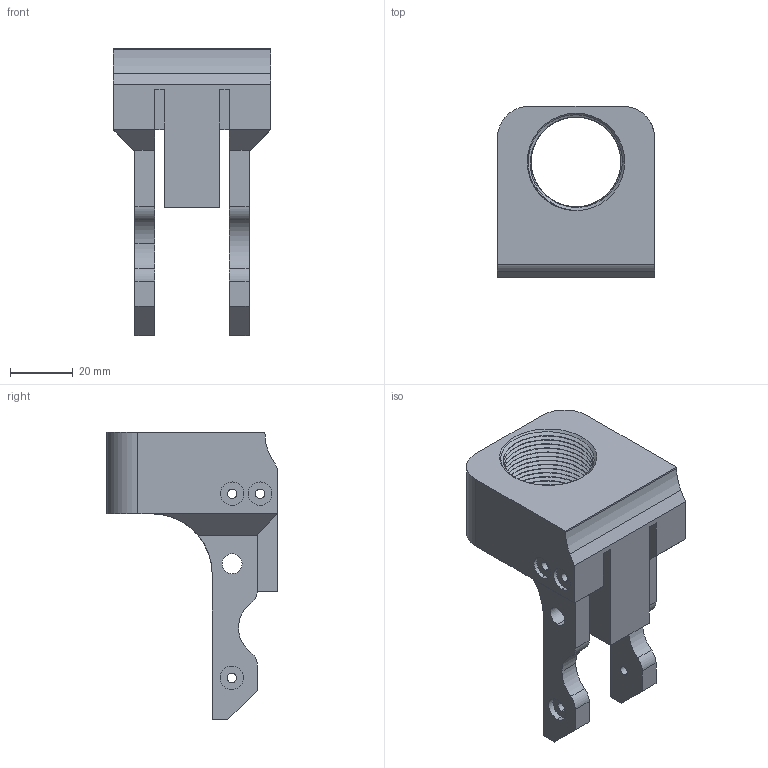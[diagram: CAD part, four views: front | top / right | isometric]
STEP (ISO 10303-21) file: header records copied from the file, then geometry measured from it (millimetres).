
FILE_DESCRIPTION (( 'STEP AP214' ), '1' );
FILE_NAME ('Reinforced_Buffer.step', '2015-06-12T17:08:53', ( '' ), ( '' ), 'SwSTEP 2.0', 'SolidWorks 2015', '' );
FILE_SCHEMA (( 'AUTOMOTIVE_DESIGN' ));
Length unit declared in the file: millimetre
Products named in the file (1): Reinforced_Buffer
Bounding box: 50 x 54.46 x 91.53 mm (x, y, z)
Volume: 64975.7 mm3; surface area: 23443.5 mm2
Topology: 1 solids, 1 shells, 208 faces, 595 edges, 394 vertices
Faces by surface type: cylinder 100, plane 60, bspline 42, cone 6
Entity records: 44973 total; most frequent: CARTESIAN_POINT 40089, ORIENTED_EDGE 1190, DIRECTION 786, EDGE_CURVE 595, VERTEX_POINT 394, AXIS2_PLACEMENT_3D 274, EDGE_LOOP 239, LINE 238
